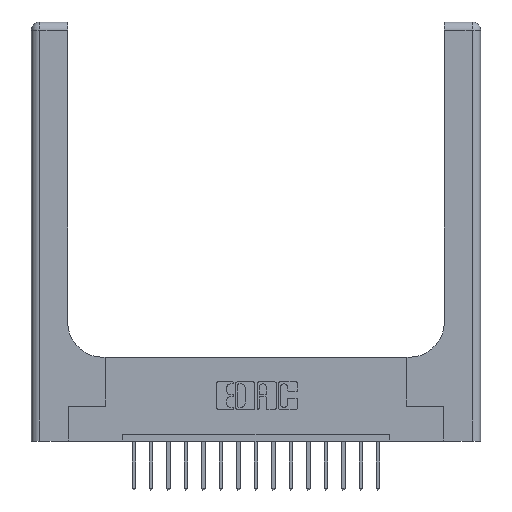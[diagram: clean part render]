
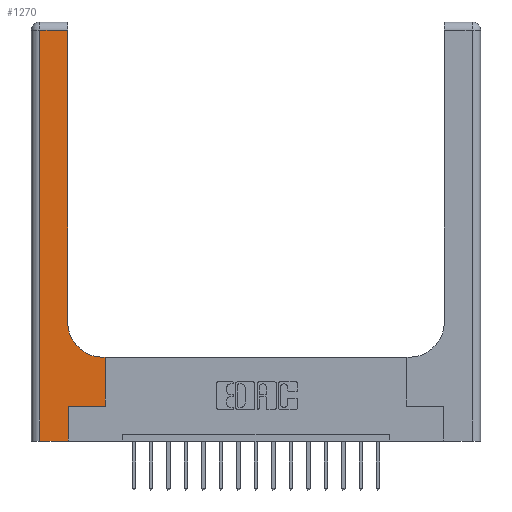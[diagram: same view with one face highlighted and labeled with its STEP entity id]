
A CAD part, top view. The second image highlights one B-rep face of the part: STEP entity #1270.
In plain terms, the highlighted planar face has unit normal (0, 0, 1).
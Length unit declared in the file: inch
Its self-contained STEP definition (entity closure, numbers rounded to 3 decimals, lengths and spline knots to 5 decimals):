
#193 = CARTESIAN_POINT ( 'NONE',  ( 0.265, 0., 0.37 ) ) ;
#281 = EDGE_CURVE ( 'NONE', #5033, #6305, #10222, .T. ) ;
#504 = EDGE_CURVE ( 'NONE', #12712, #13969, #1168, .T. ) ;
#528 = CARTESIAN_POINT ( 'NONE',  ( 0., 3., 0.37 ) ) ;
#575 = CARTESIAN_POINT ( 'NONE',  ( 0.26, 3., 0.37 ) ) ;
#658 = ORIENTED_EDGE ( 'NONE', *, *, #13088, .T. ) ;
#1020 = DIRECTION ( 'NONE',  ( 0., 1., 0. ) ) ;
#1098 = VERTEX_POINT ( 'NONE', #3050 ) ;
#1102 = VERTEX_POINT ( 'NONE', #11630 ) ;
#1168 = LINE ( 'NONE', #6845, #13073 ) ;
#1270 = ADVANCED_FACE ( 'NONE', ( #10417 ), #2098, .F. ) ;
#2040 = LINE ( 'NONE', #8083, #17405 ) ;
#2051 = CIRCLE ( 'NONE', #10989, 0.25 ) ;
#2098 = PLANE ( 'NONE',  #7996 ) ;
#2459 = EDGE_CURVE ( 'NONE', #6305, #16106, #14006, .T. ) ;
#2486 = LINE ( 'NONE', #16741, #15550 ) ;
#3050 = CARTESIAN_POINT ( 'NONE',  ( 0.528, 0.6, 0.37 ) ) ;
#3102 = EDGE_CURVE ( 'NONE', #16106, #17250, #2486, .T. ) ;
#3266 = LINE ( 'NONE', #8923, #8147 ) ;
#3390 = CARTESIAN_POINT ( 'NONE',  ( 0.528, 0.25, 0.37 ) ) ;
#3524 = VECTOR ( 'NONE', #4731, 39.37008 ) ;
#3623 = DIRECTION ( 'NONE',  ( -1., 0., 0. ) ) ;
#3667 = EDGE_CURVE ( 'NONE', #1098, #1102, #2040, .T. ) ;
#3946 = ORIENTED_EDGE ( 'NONE', *, *, #12183, .T. ) ;
#4220 = ORIENTED_EDGE ( 'NONE', *, *, #504, .T. ) ;
#4731 = DIRECTION ( 'NONE',  ( 1., 0., 0. ) ) ;
#4755 = DIRECTION ( 'NONE',  ( 0., 1., 0. ) ) ;
#4928 = DIRECTION ( 'NONE',  ( 0., 0., -1. ) ) ;
#5033 = VERTEX_POINT ( 'NONE', #9605 ) ;
#5211 = EDGE_LOOP ( 'NONE', ( #3946, #4220, #5607, #11386, #15096, #16401, #14913, #10234, #658 ) ) ;
#5213 = EDGE_CURVE ( 'NONE', #17250, #1098, #3266, .T. ) ;
#5607 = ORIENTED_EDGE ( 'NONE', *, *, #15795, .T. ) ;
#5847 = VECTOR ( 'NONE', #10720, 39.37008 ) ;
#6305 = VERTEX_POINT ( 'NONE', #193 ) ;
#6404 = DIRECTION ( 'NONE',  ( -1., 0., 0. ) ) ;
#6520 = CARTESIAN_POINT ( 'NONE',  ( 0.26, 2.94, 0.37 ) ) ;
#6706 = CARTESIAN_POINT ( 'NONE',  ( 0.265, 0., 0.37 ) ) ;
#6845 = CARTESIAN_POINT ( 'NONE',  ( 0., 2.94, 0.37 ) ) ;
#7144 = VECTOR ( 'NONE', #10377, 39.37008 ) ;
#7649 = CARTESIAN_POINT ( 'NONE',  ( 0.06, 3., 0.37 ) ) ;
#7996 = AXIS2_PLACEMENT_3D ( 'NONE', #528, #13514, #6404 ) ;
#8083 = CARTESIAN_POINT ( 'NONE',  ( 0.26, 0.6, 0.37 ) ) ;
#8147 = VECTOR ( 'NONE', #4755, 39.37008 ) ;
#8386 = CARTESIAN_POINT ( 'NONE',  ( 0.265, 0.25, 0.37 ) ) ;
#8590 = CARTESIAN_POINT ( 'NONE',  ( 0.26, 0.85, 0.37 ) ) ;
#8923 = CARTESIAN_POINT ( 'NONE',  ( 0.528, 0.25, 0.37 ) ) ;
#8953 = VERTEX_POINT ( 'NONE', #8590 ) ;
#9193 = DIRECTION ( 'NONE',  ( 1., 0., 0. ) ) ;
#9279 = CARTESIAN_POINT ( 'NONE',  ( 0.51, 0.85, 0.37 ) ) ;
#9605 = CARTESIAN_POINT ( 'NONE',  ( 0.06, 0., 0.37 ) ) ;
#10222 = LINE ( 'NONE', #17409, #3524 ) ;
#10234 = ORIENTED_EDGE ( 'NONE', *, *, #3667, .T. ) ;
#10377 = DIRECTION ( 'NONE',  ( 0., 1., 0. ) ) ;
#10417 = FACE_OUTER_BOUND ( 'NONE', #5211, .T. ) ;
#10720 = DIRECTION ( 'NONE',  ( 0., -1., 0. ) ) ;
#10989 = AXIS2_PLACEMENT_3D ( 'NONE', #9279, #4928, #9193 ) ;
#11386 = ORIENTED_EDGE ( 'NONE', *, *, #281, .T. ) ;
#11630 = CARTESIAN_POINT ( 'NONE',  ( 0.51, 0.6, 0.37 ) ) ;
#12183 = EDGE_CURVE ( 'NONE', #8953, #12712, #14611, .T. ) ;
#12552 = DIRECTION ( 'NONE',  ( 1., 0., 0. ) ) ;
#12712 = VERTEX_POINT ( 'NONE', #6520 ) ;
#13073 = VECTOR ( 'NONE', #3623, 39.37008 ) ;
#13088 = EDGE_CURVE ( 'NONE', #1102, #8953, #2051, .T. ) ;
#13286 = LINE ( 'NONE', #7649, #5847 ) ;
#13514 = DIRECTION ( 'NONE',  ( 0., 0., -1. ) ) ;
#13636 = DIRECTION ( 'NONE',  ( -1., 0., 0. ) ) ;
#13969 = VERTEX_POINT ( 'NONE', #16725 ) ;
#14006 = LINE ( 'NONE', #6706, #16739 ) ;
#14611 = LINE ( 'NONE', #575, #7144 ) ;
#14913 = ORIENTED_EDGE ( 'NONE', *, *, #5213, .T. ) ;
#15096 = ORIENTED_EDGE ( 'NONE', *, *, #2459, .T. ) ;
#15550 = VECTOR ( 'NONE', #12552, 39.37008 ) ;
#15795 = EDGE_CURVE ( 'NONE', #13969, #5033, #13286, .T. ) ;
#16106 = VERTEX_POINT ( 'NONE', #8386 ) ;
#16401 = ORIENTED_EDGE ( 'NONE', *, *, #3102, .T. ) ;
#16725 = CARTESIAN_POINT ( 'NONE',  ( 0.06, 2.94, 0.37 ) ) ;
#16739 = VECTOR ( 'NONE', #1020, 39.37008 ) ;
#16741 = CARTESIAN_POINT ( 'NONE',  ( 0.265, 0.25, 0.37 ) ) ;
#17250 = VERTEX_POINT ( 'NONE', #3390 ) ;
#17405 = VECTOR ( 'NONE', #13636, 39.37008 ) ;
#17409 = CARTESIAN_POINT ( 'NONE',  ( 0., 0., 0.37 ) ) ;
